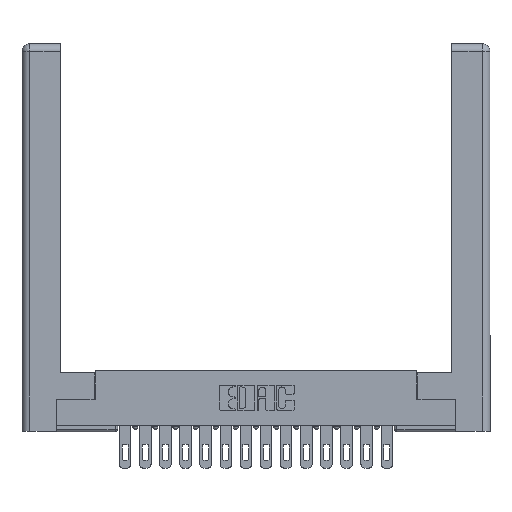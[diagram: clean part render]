
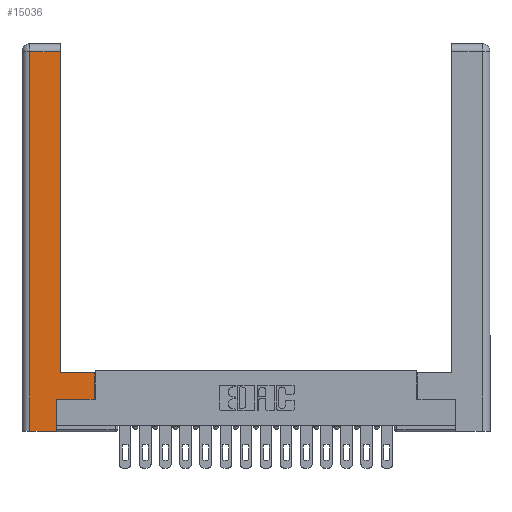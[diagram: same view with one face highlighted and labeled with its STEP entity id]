
A CAD part, top view. The second image highlights one B-rep face of the part: STEP entity #15036.
In plain terms, the highlighted planar face has unit normal (0, 0, 1).
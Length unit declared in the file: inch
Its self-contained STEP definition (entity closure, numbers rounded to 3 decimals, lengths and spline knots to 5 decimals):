
#145 = EDGE_CURVE ( 'NONE', #17266, #4598, #5321, .T. ) ;
#394 = CARTESIAN_POINT ( 'NONE',  ( 0.295, 2.94, 0. ) ) ;
#548 = DIRECTION ( 'NONE',  ( 0., 1., 0. ) ) ;
#662 = CARTESIAN_POINT ( 'NONE',  ( 0.565, 0.245, 0. ) ) ;
#743 = FACE_OUTER_BOUND ( 'NONE', #6739, .T. ) ;
#986 = VERTEX_POINT ( 'NONE', #12886 ) ;
#1288 = ORIENTED_EDGE ( 'NONE', *, *, #13248, .T. ) ;
#1349 = DIRECTION ( 'NONE',  ( 0., -1., 0. ) ) ;
#1450 = VECTOR ( 'NONE', #4158, 39.37008 ) ;
#1458 = ORIENTED_EDGE ( 'NONE', *, *, #12231, .T. ) ;
#2347 = CARTESIAN_POINT ( 'NONE',  ( 0.265, 0., 0. ) ) ;
#2529 = CARTESIAN_POINT ( 'NONE',  ( 0., 0., 0. ) ) ;
#2577 = VERTEX_POINT ( 'NONE', #662 ) ;
#2594 = DIRECTION ( 'NONE',  ( 0., 0., -1. ) ) ;
#3774 = ORIENTED_EDGE ( 'NONE', *, *, #16191, .T. ) ;
#4158 = DIRECTION ( 'NONE',  ( 1., 0., 0. ) ) ;
#4206 = VECTOR ( 'NONE', #8808, 39.37008 ) ;
#4598 = VERTEX_POINT ( 'NONE', #4783 ) ;
#4783 = CARTESIAN_POINT ( 'NONE',  ( 0.0615, 2.94, 0. ) ) ;
#4931 = ORIENTED_EDGE ( 'NONE', *, *, #145, .T. ) ;
#5216 = DIRECTION ( 'NONE',  ( 1., 0., 0. ) ) ;
#5321 = LINE ( 'NONE', #8836, #7087 ) ;
#5418 = VERTEX_POINT ( 'NONE', #18141 ) ;
#5928 = CARTESIAN_POINT ( 'NONE',  ( 0.295, 3., 0. ) ) ;
#5997 = LINE ( 'NONE', #11249, #4206 ) ;
#6659 = VECTOR ( 'NONE', #1349, 39.37008 ) ;
#6739 = EDGE_LOOP ( 'NONE', ( #3774, #4931, #1458, #7664, #7753, #12487, #10771, #1288 ) ) ;
#7087 = VECTOR ( 'NONE', #13342, 39.37008 ) ;
#7454 = LINE ( 'NONE', #8465, #1450 ) ;
#7664 = ORIENTED_EDGE ( 'NONE', *, *, #10086, .T. ) ;
#7753 = ORIENTED_EDGE ( 'NONE', *, *, #18408, .T. ) ;
#7975 = LINE ( 'NONE', #13835, #6659 ) ;
#8001 = AXIS2_PLACEMENT_3D ( 'NONE', #2529, #2594, #12515 ) ;
#8465 = CARTESIAN_POINT ( 'NONE',  ( 0.565, 0.245, 0. ) ) ;
#8808 = DIRECTION ( 'NONE',  ( 0., 1., 0. ) ) ;
#8836 = CARTESIAN_POINT ( 'NONE',  ( 0.0615, 2.94, 0. ) ) ;
#8860 = EDGE_CURVE ( 'NONE', #12821, #2577, #7454, .T. ) ;
#9035 = DIRECTION ( 'NONE',  ( 0., 1., 0. ) ) ;
#9203 = CARTESIAN_POINT ( 'NONE',  ( 0.295, 0.45, 0. ) ) ;
#10086 = EDGE_CURVE ( 'NONE', #12817, #11364, #15669, .T. ) ;
#10771 = ORIENTED_EDGE ( 'NONE', *, *, #17715, .T. ) ;
#11055 = VECTOR ( 'NONE', #16322, 39.37008 ) ;
#11194 = VECTOR ( 'NONE', #548, 39.37008 ) ;
#11249 = CARTESIAN_POINT ( 'NONE',  ( 0.565, 0.45, 0. ) ) ;
#11364 = VERTEX_POINT ( 'NONE', #12369 ) ;
#12231 = EDGE_CURVE ( 'NONE', #4598, #12817, #7975, .T. ) ;
#12369 = CARTESIAN_POINT ( 'NONE',  ( 0.265, 0., 0. ) ) ;
#12487 = ORIENTED_EDGE ( 'NONE', *, *, #8860, .T. ) ;
#12515 = DIRECTION ( 'NONE',  ( -1., 0., 0. ) ) ;
#12817 = VERTEX_POINT ( 'NONE', #15735 ) ;
#12821 = VERTEX_POINT ( 'NONE', #14482 ) ;
#12886 = CARTESIAN_POINT ( 'NONE',  ( 0.565, 0.45, 0. ) ) ;
#13234 = VECTOR ( 'NONE', #5216, 39.37008 ) ;
#13248 = EDGE_CURVE ( 'NONE', #986, #5418, #14851, .T. ) ;
#13342 = DIRECTION ( 'NONE',  ( -1., 0., 0. ) ) ;
#13419 = CARTESIAN_POINT ( 'NONE',  ( 0.265, 0.245, 0. ) ) ;
#13835 = CARTESIAN_POINT ( 'NONE',  ( 0.0615, 0., 0. ) ) ;
#14482 = CARTESIAN_POINT ( 'NONE',  ( 0.265, 0.245, 0. ) ) ;
#14851 = LINE ( 'NONE', #9203, #11055 ) ;
#15036 = ADVANCED_FACE ( 'NONE', ( #743 ), #16755, .F. ) ;
#15669 = LINE ( 'NONE', #2347, #13234 ) ;
#15735 = CARTESIAN_POINT ( 'NONE',  ( 0.0615, 0., 0. ) ) ;
#16032 = LINE ( 'NONE', #13419, #16694 ) ;
#16191 = EDGE_CURVE ( 'NONE', #5418, #17266, #17892, .T. ) ;
#16322 = DIRECTION ( 'NONE',  ( -1., 0., 0. ) ) ;
#16694 = VECTOR ( 'NONE', #9035, 39.37008 ) ;
#16755 = PLANE ( 'NONE',  #8001 ) ;
#17266 = VERTEX_POINT ( 'NONE', #394 ) ;
#17715 = EDGE_CURVE ( 'NONE', #2577, #986, #5997, .T. ) ;
#17892 = LINE ( 'NONE', #5928, #11194 ) ;
#18141 = CARTESIAN_POINT ( 'NONE',  ( 0.295, 0.45, 0. ) ) ;
#18408 = EDGE_CURVE ( 'NONE', #11364, #12821, #16032, .T. ) ;
